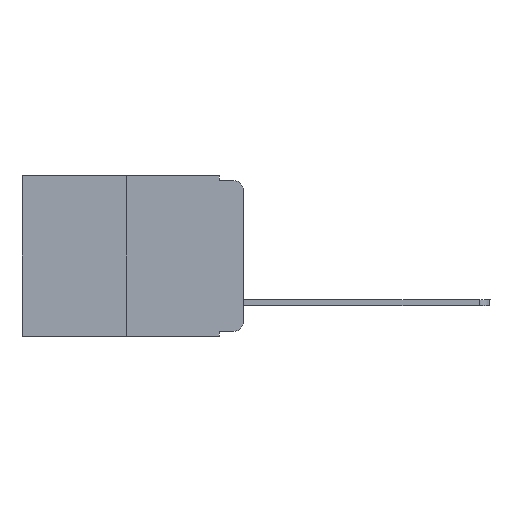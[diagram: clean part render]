
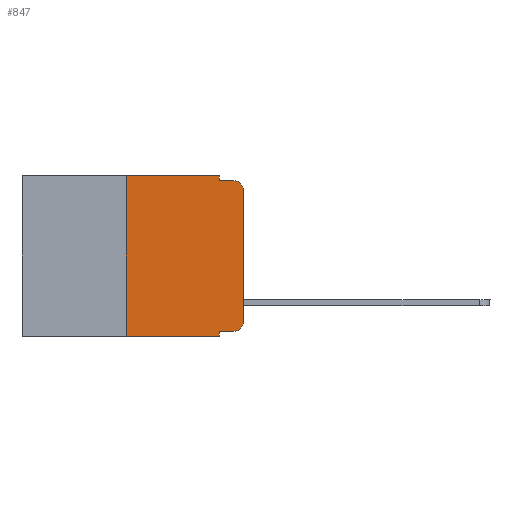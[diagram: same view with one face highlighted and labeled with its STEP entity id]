
A CAD part, left-side view. The second image highlights one B-rep face of the part: STEP entity #847.
In plain terms, the highlighted planar face has unit normal (-1, 0, 0).
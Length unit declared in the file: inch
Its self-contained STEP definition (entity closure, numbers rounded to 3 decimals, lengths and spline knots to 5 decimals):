
#14 = CARTESIAN_POINT ( 'NONE',  ( 0., 0.25, 0. ) ) ;
#166 = PLANE ( 'NONE',  #6655 ) ;
#263 = ORIENTED_EDGE ( 'NONE', *, *, #2499, .T. ) ;
#388 = LINE ( 'NONE', #7756, #3985 ) ;
#399 = AXIS2_PLACEMENT_3D ( 'NONE', #5184, #1503, #6689 ) ;
#529 = CARTESIAN_POINT ( 'NONE',  ( 0., 0.02, -0.01 ) ) ;
#620 = LINE ( 'NONE', #5181, #1897 ) ;
#702 = DIRECTION ( 'NONE',  ( 0., 0., -1. ) ) ;
#833 = FACE_OUTER_BOUND ( 'NONE', #1396, .T. ) ;
#847 = ADVANCED_FACE ( 'NONE', ( #833 ), #166, .F. ) ;
#1047 = DIRECTION ( 'NONE',  ( 0., 0., -1. ) ) ;
#1101 = CARTESIAN_POINT ( 'NONE',  ( 0., 0.051, -0.333 ) ) ;
#1231 = CARTESIAN_POINT ( 'NONE',  ( 0., 0.051, -0.333 ) ) ;
#1332 = CARTESIAN_POINT ( 'NONE',  ( 0., 0.051, -0.01 ) ) ;
#1356 = VERTEX_POINT ( 'NONE', #5895 ) ;
#1396 = EDGE_LOOP ( 'NONE', ( #1507, #6229, #8971, #5008, #3703, #1726, #1480, #2592, #263, #5961 ) ) ;
#1480 = ORIENTED_EDGE ( 'NONE', *, *, #6816, .T. ) ;
#1503 = DIRECTION ( 'NONE',  ( -1., 0., 0. ) ) ;
#1507 = ORIENTED_EDGE ( 'NONE', *, *, #2164, .T. ) ;
#1687 = CARTESIAN_POINT ( 'NONE',  ( 0., 0.473, 0. ) ) ;
#1726 = ORIENTED_EDGE ( 'NONE', *, *, #7422, .F. ) ;
#1793 = LINE ( 'NONE', #4754, #3202 ) ;
#1884 = VERTEX_POINT ( 'NONE', #7602 ) ;
#1897 = VECTOR ( 'NONE', #8033, 39.37008 ) ;
#2116 = DIRECTION ( 'NONE',  ( 0., -1., 0. ) ) ;
#2164 = EDGE_CURVE ( 'NONE', #1356, #2256, #620, .T. ) ;
#2256 = VERTEX_POINT ( 'NONE', #7496 ) ;
#2263 = CIRCLE ( 'NONE', #399, 0.02 ) ;
#2385 = VERTEX_POINT ( 'NONE', #7165 ) ;
#2441 = VECTOR ( 'NONE', #5756, 39.37008 ) ;
#2499 = EDGE_CURVE ( 'NONE', #3109, #1884, #4943, .T. ) ;
#2592 = ORIENTED_EDGE ( 'NONE', *, *, #5806, .F. ) ;
#2612 = EDGE_CURVE ( 'NONE', #2385, #3246, #7528, .T. ) ;
#2669 = DIRECTION ( 'NONE',  ( 0., 0., -1. ) ) ;
#2710 = CARTESIAN_POINT ( 'NONE',  ( 0., 0.473, 0. ) ) ;
#2830 = LINE ( 'NONE', #9415, #2441 ) ;
#2967 = DIRECTION ( 'NONE',  ( 0., 0., 1. ) ) ;
#3066 = CARTESIAN_POINT ( 'NONE',  ( 0., 0.25, 0. ) ) ;
#3109 = VERTEX_POINT ( 'NONE', #1101 ) ;
#3202 = VECTOR ( 'NONE', #1047, 39.37008 ) ;
#3246 = VERTEX_POINT ( 'NONE', #529 ) ;
#3703 = ORIENTED_EDGE ( 'NONE', *, *, #4645, .F. ) ;
#3718 = DIRECTION ( 'NONE',  ( 1., 0., 0. ) ) ;
#3765 = VECTOR ( 'NONE', #4164, 39.37008 ) ;
#3985 = VECTOR ( 'NONE', #2669, 39.37008 ) ;
#4114 = VECTOR ( 'NONE', #2967, 39.37008 ) ;
#4164 = DIRECTION ( 'NONE',  ( 0., -1., 0. ) ) ;
#4401 = CARTESIAN_POINT ( 'NONE',  ( 0., 0.02, -0.313 ) ) ;
#4645 = EDGE_CURVE ( 'NONE', #5731, #7637, #9474, .T. ) ;
#4754 = CARTESIAN_POINT ( 'NONE',  ( 0., 0.051, 0. ) ) ;
#4859 = EDGE_CURVE ( 'NONE', #2256, #3246, #2263, .T. ) ;
#4943 = LINE ( 'NONE', #1231, #3765 ) ;
#5008 = ORIENTED_EDGE ( 'NONE', *, *, #9101, .F. ) ;
#5181 = CARTESIAN_POINT ( 'NONE',  ( 0., 0., 0. ) ) ;
#5184 = CARTESIAN_POINT ( 'NONE',  ( 0., 0.02, -0.03 ) ) ;
#5279 = EDGE_CURVE ( 'NONE', #1884, #1356, #8140, .T. ) ;
#5497 = CARTESIAN_POINT ( 'NONE',  ( 0., 0.25, -0.343 ) ) ;
#5731 = VERTEX_POINT ( 'NONE', #3066 ) ;
#5756 = DIRECTION ( 'NONE',  ( 0., -1., 0. ) ) ;
#5774 = CARTESIAN_POINT ( 'NONE',  ( 0., 0.051, 0. ) ) ;
#5806 = EDGE_CURVE ( 'NONE', #3109, #8281, #388, .T. ) ;
#5895 = CARTESIAN_POINT ( 'NONE',  ( 0., 0., -0.313 ) ) ;
#5961 = ORIENTED_EDGE ( 'NONE', *, *, #5279, .T. ) ;
#6195 = CARTESIAN_POINT ( 'NONE',  ( 0., 0.051, -0.343 ) ) ;
#6229 = ORIENTED_EDGE ( 'NONE', *, *, #4859, .T. ) ;
#6655 = AXIS2_PLACEMENT_3D ( 'NONE', #1687, #3718, #8110 ) ;
#6658 = LINE ( 'NONE', #14, #4114 ) ;
#6689 = DIRECTION ( 'NONE',  ( 0., 0., -1. ) ) ;
#6816 = EDGE_CURVE ( 'NONE', #8828, #8281, #2830, .T. ) ;
#6940 = VECTOR ( 'NONE', #9430, 39.37008 ) ;
#7165 = CARTESIAN_POINT ( 'NONE',  ( 0., 0.051, -0.01 ) ) ;
#7348 = DIRECTION ( 'NONE',  ( -1., 0., 0. ) ) ;
#7422 = EDGE_CURVE ( 'NONE', #8828, #5731, #6658, .T. ) ;
#7496 = CARTESIAN_POINT ( 'NONE',  ( 0., 0., -0.03 ) ) ;
#7528 = LINE ( 'NONE', #1332, #9316 ) ;
#7602 = CARTESIAN_POINT ( 'NONE',  ( 0., 0.02, -0.333 ) ) ;
#7637 = VERTEX_POINT ( 'NONE', #5774 ) ;
#7756 = CARTESIAN_POINT ( 'NONE',  ( 0., 0.051, 0. ) ) ;
#8033 = DIRECTION ( 'NONE',  ( 0., 0., 1. ) ) ;
#8110 = DIRECTION ( 'NONE',  ( 0., 0., -1. ) ) ;
#8140 = CIRCLE ( 'NONE', #8602, 0.02 ) ;
#8281 = VERTEX_POINT ( 'NONE', #6195 ) ;
#8602 = AXIS2_PLACEMENT_3D ( 'NONE', #4401, #7348, #702 ) ;
#8828 = VERTEX_POINT ( 'NONE', #5497 ) ;
#8971 = ORIENTED_EDGE ( 'NONE', *, *, #2612, .F. ) ;
#9101 = EDGE_CURVE ( 'NONE', #7637, #2385, #1793, .T. ) ;
#9316 = VECTOR ( 'NONE', #2116, 39.37008 ) ;
#9415 = CARTESIAN_POINT ( 'NONE',  ( 0., 0.473, -0.343 ) ) ;
#9430 = DIRECTION ( 'NONE',  ( 0., -1., 0. ) ) ;
#9474 = LINE ( 'NONE', #2710, #6940 ) ;
